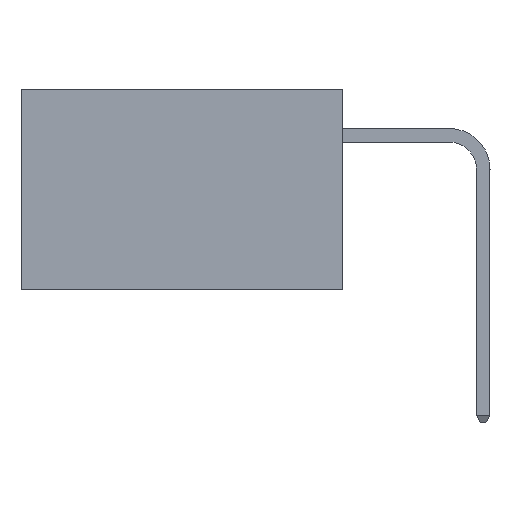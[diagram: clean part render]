
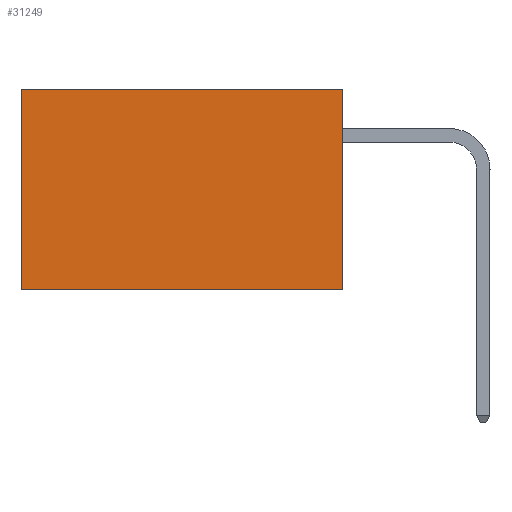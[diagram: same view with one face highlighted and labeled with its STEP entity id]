
A CAD part, left-side view. The second image highlights one B-rep face of the part: STEP entity #31249.
In plain terms, the highlighted planar face has unit normal (-1, 0, 0).
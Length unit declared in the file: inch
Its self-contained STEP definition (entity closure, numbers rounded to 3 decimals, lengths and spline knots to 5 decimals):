
#1771 = ORIENTED_EDGE ( 'NONE', *, *, #11194, .T. ) ;
#3259 = VECTOR ( 'NONE', #12328, 39.37008 ) ;
#5017 = CARTESIAN_POINT ( 'NONE',  ( 0.277, 0.59, 0. ) ) ;
#5018 = EDGE_LOOP ( 'NONE', ( #1771, #26842, #16145, #30726 ) ) ;
#6786 = CARTESIAN_POINT ( 'NONE',  ( 0.277, 0.59, -0.37 ) ) ;
#7083 = VERTEX_POINT ( 'NONE', #23454 ) ;
#7317 = EDGE_CURVE ( 'NONE', #23156, #7083, #10106, .T. ) ;
#10106 = LINE ( 'NONE', #13413, #3259 ) ;
#10370 = CARTESIAN_POINT ( 'NONE',  ( 0.277, 0., 0. ) ) ;
#11194 = EDGE_CURVE ( 'NONE', #30292, #25806, #27272, .T. ) ;
#11401 = DIRECTION ( 'NONE',  ( 0., 1., 0. ) ) ;
#12328 = DIRECTION ( 'NONE',  ( 0., 0., -1. ) ) ;
#12422 = CARTESIAN_POINT ( 'NONE',  ( 0.277, 0., -0.37 ) ) ;
#13191 = VECTOR ( 'NONE', #22941, 39.37008 ) ;
#13413 = CARTESIAN_POINT ( 'NONE',  ( 0.277, 0., -0.37 ) ) ;
#13426 = PLANE ( 'NONE',  #16276 ) ;
#13596 = EDGE_CURVE ( 'NONE', #7083, #25806, #21341, .T. ) ;
#15785 = LINE ( 'NONE', #21462, #28241 ) ;
#15954 = DIRECTION ( 'NONE',  ( 0., 0., -1. ) ) ;
#16145 = ORIENTED_EDGE ( 'NONE', *, *, #7317, .F. ) ;
#16276 = AXIS2_PLACEMENT_3D ( 'NONE', #28345, #30792, #15954 ) ;
#20574 = VECTOR ( 'NONE', #22440, 39.37008 ) ;
#20969 = EDGE_CURVE ( 'NONE', #23156, #30292, #15785, .T. ) ;
#21341 = LINE ( 'NONE', #12422, #20574 ) ;
#21462 = CARTESIAN_POINT ( 'NONE',  ( 0.277, 0., 0. ) ) ;
#22440 = DIRECTION ( 'NONE',  ( 0., 1., 0. ) ) ;
#22941 = DIRECTION ( 'NONE',  ( 0., 0., -1. ) ) ;
#23003 = CARTESIAN_POINT ( 'NONE',  ( 0.277, 0.59, -0.37 ) ) ;
#23156 = VERTEX_POINT ( 'NONE', #10370 ) ;
#23454 = CARTESIAN_POINT ( 'NONE',  ( 0.277, 0., -0.37 ) ) ;
#24691 = FACE_OUTER_BOUND ( 'NONE', #5018, .T. ) ;
#25806 = VERTEX_POINT ( 'NONE', #6786 ) ;
#26842 = ORIENTED_EDGE ( 'NONE', *, *, #13596, .F. ) ;
#27272 = LINE ( 'NONE', #23003, #13191 ) ;
#28241 = VECTOR ( 'NONE', #11401, 39.37008 ) ;
#28345 = CARTESIAN_POINT ( 'NONE',  ( 0.277, 0., -0.37 ) ) ;
#30292 = VERTEX_POINT ( 'NONE', #5017 ) ;
#30726 = ORIENTED_EDGE ( 'NONE', *, *, #20969, .T. ) ;
#30792 = DIRECTION ( 'NONE',  ( 1., 0., 0. ) ) ;
#31249 = ADVANCED_FACE ( 'NONE', ( #24691 ), #13426, .F. ) ;
